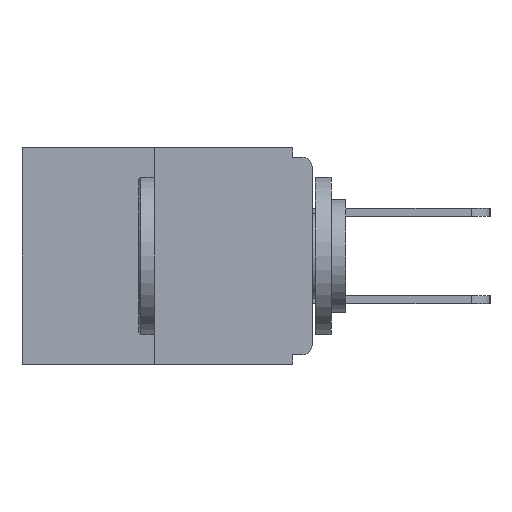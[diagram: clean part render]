
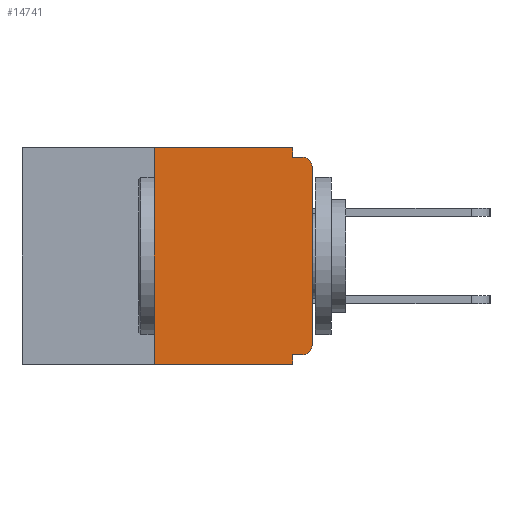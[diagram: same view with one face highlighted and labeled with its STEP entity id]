
A CAD part, left-side view. The second image highlights one B-rep face of the part: STEP entity #14741.
In plain terms, the highlighted planar face has unit normal (-1, 0, 0).
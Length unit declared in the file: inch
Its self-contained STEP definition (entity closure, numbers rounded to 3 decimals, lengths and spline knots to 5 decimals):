
#114 = EDGE_CURVE ( 'NONE', #20327, #1764, #8505, .T. ) ;
#264 = ORIENTED_EDGE ( 'NONE', *, *, #1348, .T. ) ;
#268 = VERTEX_POINT ( 'NONE', #1425 ) ;
#601 = EDGE_CURVE ( 'NONE', #16193, #268, #4986, .T. ) ;
#609 = ORIENTED_EDGE ( 'NONE', *, *, #11636, .F. ) ;
#814 = VERTEX_POINT ( 'NONE', #6480 ) ;
#1348 = EDGE_CURVE ( 'NONE', #16193, #21545, #21317, .T. ) ;
#1425 = CARTESIAN_POINT ( 'NONE',  ( 0., 0.031, -0.328 ) ) ;
#1472 = LINE ( 'NONE', #12765, #15330 ) ;
#1610 = VECTOR ( 'NONE', #19949, 39.37008 ) ;
#1711 = AXIS2_PLACEMENT_3D ( 'NONE', #4916, #11949, #3408 ) ;
#1764 = VERTEX_POINT ( 'NONE', #15817 ) ;
#3011 = AXIS2_PLACEMENT_3D ( 'NONE', #13020, #18278, #16513 ) ;
#3179 = PLANE ( 'NONE',  #1711 ) ;
#3408 = DIRECTION ( 'NONE',  ( 0., 0., -1. ) ) ;
#4125 = ORIENTED_EDGE ( 'NONE', *, *, #6134, .T. ) ;
#4200 = CARTESIAN_POINT ( 'NONE',  ( 0., 0.031, -0.343 ) ) ;
#4496 = DIRECTION ( 'NONE',  ( -1., 0., 0. ) ) ;
#4796 = CARTESIAN_POINT ( 'NONE',  ( 0., 0.015, -0.328 ) ) ;
#4916 = CARTESIAN_POINT ( 'NONE',  ( 0., 0.46, 0. ) ) ;
#4986 = LINE ( 'NONE', #12551, #17492 ) ;
#5163 = EDGE_CURVE ( 'NONE', #814, #10720, #22522, .T. ) ;
#5206 = ORIENTED_EDGE ( 'NONE', *, *, #6803, .F. ) ;
#5278 = CARTESIAN_POINT ( 'NONE',  ( 0., 0.031, -0.343 ) ) ;
#6134 = EDGE_CURVE ( 'NONE', #21545, #20327, #12887, .T. ) ;
#6218 = DIRECTION ( 'NONE',  ( 0., 0., -1. ) ) ;
#6480 = CARTESIAN_POINT ( 'NONE',  ( 0., 0.25, -0.343 ) ) ;
#6803 = EDGE_CURVE ( 'NONE', #13424, #22467, #1472, .T. ) ;
#7502 = LINE ( 'NONE', #16646, #15425 ) ;
#7761 = ORIENTED_EDGE ( 'NONE', *, *, #10685, .F. ) ;
#7776 = EDGE_CURVE ( 'NONE', #22467, #1764, #13352, .T. ) ;
#8065 = ORIENTED_EDGE ( 'NONE', *, *, #5163, .F. ) ;
#8505 = CIRCLE ( 'NONE', #13606, 0.015 ) ;
#8572 = DIRECTION ( 'NONE',  ( 0., -1., 0. ) ) ;
#9495 = FACE_OUTER_BOUND ( 'NONE', #19444, .T. ) ;
#9527 = CARTESIAN_POINT ( 'NONE',  ( 0., 0.25, 0. ) ) ;
#10685 = EDGE_CURVE ( 'NONE', #268, #17160, #17651, .T. ) ;
#10720 = VERTEX_POINT ( 'NONE', #9527 ) ;
#11447 = DIRECTION ( 'NONE',  ( 0., 0., 1. ) ) ;
#11636 = EDGE_CURVE ( 'NONE', #10720, #13424, #7502, .T. ) ;
#11710 = VECTOR ( 'NONE', #13267, 39.37008 ) ;
#11924 = CARTESIAN_POINT ( 'NONE',  ( 0., 0.46, -0.343 ) ) ;
#11949 = DIRECTION ( 'NONE',  ( 1., 0., 0. ) ) ;
#12551 = CARTESIAN_POINT ( 'NONE',  ( 0., 0., -0.328 ) ) ;
#12765 = CARTESIAN_POINT ( 'NONE',  ( 0., 0.031, 0. ) ) ;
#12812 = CARTESIAN_POINT ( 'NONE',  ( 0., 0., 0. ) ) ;
#12887 = LINE ( 'NONE', #12812, #20318 ) ;
#12994 = DIRECTION ( 'NONE',  ( 0., -1., 0. ) ) ;
#13020 = CARTESIAN_POINT ( 'NONE',  ( 0., 0.015, -0.313 ) ) ;
#13267 = DIRECTION ( 'NONE',  ( 0., -1., 0. ) ) ;
#13352 = LINE ( 'NONE', #18758, #11710 ) ;
#13424 = VERTEX_POINT ( 'NONE', #18490 ) ;
#13606 = AXIS2_PLACEMENT_3D ( 'NONE', #21877, #4496, #6218 ) ;
#14594 = DIRECTION ( 'NONE',  ( 0., 0., -1. ) ) ;
#14682 = CARTESIAN_POINT ( 'NONE',  ( 0., 0.031, -0.015 ) ) ;
#14741 = ADVANCED_FACE ( 'NONE', ( #9495 ), #3179, .F. ) ;
#15330 = VECTOR ( 'NONE', #14594, 39.37008 ) ;
#15425 = VECTOR ( 'NONE', #12994, 39.37008 ) ;
#15817 = CARTESIAN_POINT ( 'NONE',  ( 0., 0.015, -0.015 ) ) ;
#16071 = VECTOR ( 'NONE', #8572, 39.37008 ) ;
#16193 = VERTEX_POINT ( 'NONE', #4796 ) ;
#16513 = DIRECTION ( 'NONE',  ( 0., 0., -1. ) ) ;
#16646 = CARTESIAN_POINT ( 'NONE',  ( 0., 0.46, 0. ) ) ;
#16933 = ORIENTED_EDGE ( 'NONE', *, *, #7776, .F. ) ;
#17160 = VERTEX_POINT ( 'NONE', #5278 ) ;
#17189 = LINE ( 'NONE', #11924, #16071 ) ;
#17492 = VECTOR ( 'NONE', #19585, 39.37008 ) ;
#17651 = LINE ( 'NONE', #4200, #1610 ) ;
#18278 = DIRECTION ( 'NONE',  ( -1., 0., 0. ) ) ;
#18490 = CARTESIAN_POINT ( 'NONE',  ( 0., 0.031, 0. ) ) ;
#18688 = CARTESIAN_POINT ( 'NONE',  ( 0., 0., -0.03 ) ) ;
#18758 = CARTESIAN_POINT ( 'NONE',  ( 0., 0., -0.015 ) ) ;
#18992 = ORIENTED_EDGE ( 'NONE', *, *, #114, .T. ) ;
#19442 = ORIENTED_EDGE ( 'NONE', *, *, #601, .F. ) ;
#19444 = EDGE_LOOP ( 'NONE', ( #609, #8065, #21061, #7761, #19442, #264, #4125, #18992, #16933, #5206 ) ) ;
#19585 = DIRECTION ( 'NONE',  ( 0., 1., 0. ) ) ;
#19949 = DIRECTION ( 'NONE',  ( 0., 0., -1. ) ) ;
#20318 = VECTOR ( 'NONE', #21475, 39.37008 ) ;
#20327 = VERTEX_POINT ( 'NONE', #18688 ) ;
#20422 = CARTESIAN_POINT ( 'NONE',  ( 0., 0., -0.313 ) ) ;
#20472 = EDGE_CURVE ( 'NONE', #814, #17160, #17189, .T. ) ;
#21061 = ORIENTED_EDGE ( 'NONE', *, *, #20472, .T. ) ;
#21317 = CIRCLE ( 'NONE', #3011, 0.015 ) ;
#21475 = DIRECTION ( 'NONE',  ( 0., 0., 1. ) ) ;
#21545 = VERTEX_POINT ( 'NONE', #20422 ) ;
#21572 = CARTESIAN_POINT ( 'NONE',  ( 0., 0.25, 0. ) ) ;
#21708 = VECTOR ( 'NONE', #11447, 39.37008 ) ;
#21877 = CARTESIAN_POINT ( 'NONE',  ( 0., 0.015, -0.03 ) ) ;
#22467 = VERTEX_POINT ( 'NONE', #14682 ) ;
#22522 = LINE ( 'NONE', #21572, #21708 ) ;
